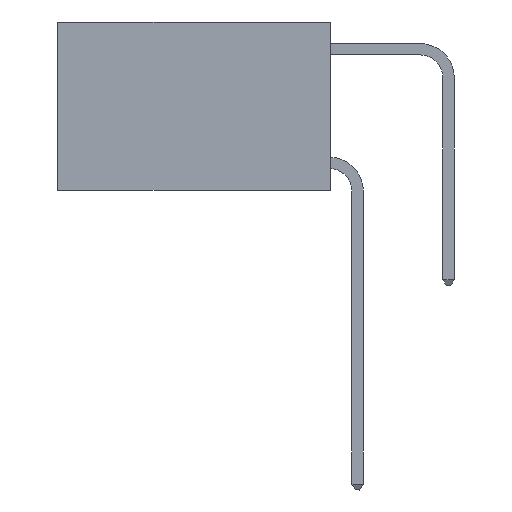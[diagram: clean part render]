
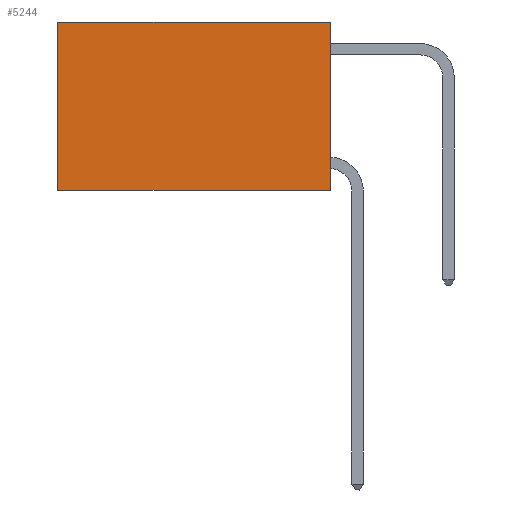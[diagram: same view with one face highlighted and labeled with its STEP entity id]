
A CAD part, left-side view. The second image highlights one B-rep face of the part: STEP entity #5244.
In plain terms, the highlighted planar face has unit normal (-1, 0, 0).
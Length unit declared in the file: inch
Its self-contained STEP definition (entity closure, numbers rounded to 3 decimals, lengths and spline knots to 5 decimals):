
#72 = PLANE ( 'NONE',  #11241 ) ;
#419 = LINE ( 'NONE', #6862, #10388 ) ;
#637 = EDGE_LOOP ( 'NONE', ( #2453, #10664, #5250, #6473 ) ) ;
#654 = LINE ( 'NONE', #12079, #8187 ) ;
#817 = VERTEX_POINT ( 'NONE', #8094 ) ;
#2074 = DIRECTION ( 'NONE',  ( 1., 0., 0. ) ) ;
#2169 = DIRECTION ( 'NONE',  ( 0., 1., 0. ) ) ;
#2453 = ORIENTED_EDGE ( 'NONE', *, *, #9913, .T. ) ;
#2908 = CARTESIAN_POINT ( 'NONE',  ( 0.2625, 0., -0.37 ) ) ;
#3098 = VERTEX_POINT ( 'NONE', #12191 ) ;
#5244 = ADVANCED_FACE ( 'NONE', ( #9671 ), #72, .F. ) ;
#5250 = ORIENTED_EDGE ( 'NONE', *, *, #5797, .F. ) ;
#5797 = EDGE_CURVE ( 'NONE', #9155, #817, #419, .T. ) ;
#5877 = DIRECTION ( 'NONE',  ( 0., 0., -1. ) ) ;
#6223 = CARTESIAN_POINT ( 'NONE',  ( 0.2625, 0., 0. ) ) ;
#6473 = ORIENTED_EDGE ( 'NONE', *, *, #8477, .T. ) ;
#6741 = VECTOR ( 'NONE', #2169, 39.37008 ) ;
#6862 = CARTESIAN_POINT ( 'NONE',  ( 0.2625, 0., 0. ) ) ;
#6975 = CARTESIAN_POINT ( 'NONE',  ( 0.2625, 0.6, -0.37 ) ) ;
#7187 = LINE ( 'NONE', #8625, #9062 ) ;
#8069 = DIRECTION ( 'NONE',  ( 0., 0., -1. ) ) ;
#8094 = CARTESIAN_POINT ( 'NONE',  ( 0.2625, 0., -0.37 ) ) ;
#8187 = VECTOR ( 'NONE', #12207, 39.37008 ) ;
#8332 = DIRECTION ( 'NONE',  ( 0., 1., 0. ) ) ;
#8477 = EDGE_CURVE ( 'NONE', #9155, #3098, #7187, .T. ) ;
#8625 = CARTESIAN_POINT ( 'NONE',  ( 0.2625, 0., 0. ) ) ;
#9062 = VECTOR ( 'NONE', #8332, 39.37008 ) ;
#9155 = VERTEX_POINT ( 'NONE', #6223 ) ;
#9204 = LINE ( 'NONE', #2908, #6741 ) ;
#9545 = EDGE_CURVE ( 'NONE', #817, #11716, #9204, .T. ) ;
#9671 = FACE_OUTER_BOUND ( 'NONE', #637, .T. ) ;
#9913 = EDGE_CURVE ( 'NONE', #3098, #11716, #654, .T. ) ;
#10388 = VECTOR ( 'NONE', #8069, 39.37008 ) ;
#10598 = CARTESIAN_POINT ( 'NONE',  ( 0.2625, 0., 0. ) ) ;
#10664 = ORIENTED_EDGE ( 'NONE', *, *, #9545, .F. ) ;
#11241 = AXIS2_PLACEMENT_3D ( 'NONE', #10598, #2074, #5877 ) ;
#11716 = VERTEX_POINT ( 'NONE', #6975 ) ;
#12079 = CARTESIAN_POINT ( 'NONE',  ( 0.2625, 0.6, 0. ) ) ;
#12191 = CARTESIAN_POINT ( 'NONE',  ( 0.2625, 0.6, 0. ) ) ;
#12207 = DIRECTION ( 'NONE',  ( 0., 0., -1. ) ) ;
